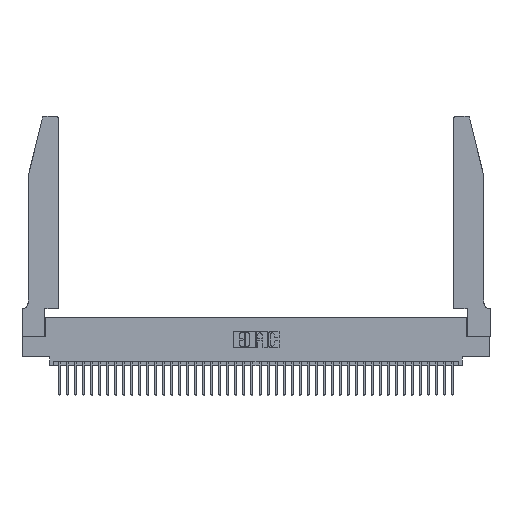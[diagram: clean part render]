
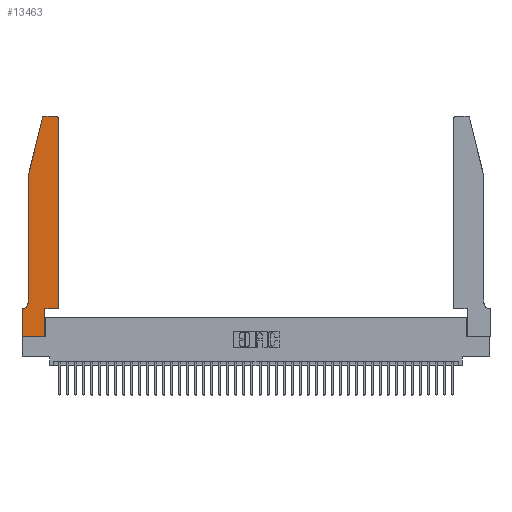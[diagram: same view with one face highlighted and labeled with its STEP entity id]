
A CAD part, top view. The second image highlights one B-rep face of the part: STEP entity #13463.
In plain terms, the highlighted planar face has unit normal (0, 0, 1).
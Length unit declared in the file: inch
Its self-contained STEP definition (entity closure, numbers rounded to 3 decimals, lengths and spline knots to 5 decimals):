
#49 = LINE ( 'NONE', #21602, #2139 ) ;
#389 = AXIS2_PLACEMENT_3D ( 'NONE', #16383, #23468, #19824 ) ;
#739 = CARTESIAN_POINT ( 'NONE',  ( 0.284, 2.75, 0.37 ) ) ;
#1626 = ORIENTED_EDGE ( 'NONE', *, *, #38126, .T. ) ;
#1852 = DIRECTION ( 'NONE',  ( 0., 1., 0. ) ) ;
#2139 = VECTOR ( 'NONE', #38475, 39.37008 ) ;
#2283 = EDGE_CURVE ( 'NONE', #10870, #23403, #25872, .T. ) ;
#2323 = VERTEX_POINT ( 'NONE', #41332 ) ;
#3364 = DIRECTION ( 'NONE',  ( 0., 0., 1. ) ) ;
#3447 = VECTOR ( 'NONE', #32906, 39.37008 ) ;
#3657 = CARTESIAN_POINT ( 'NONE',  ( 0.25487, 2.72718, 0.37 ) ) ;
#4674 = VERTEX_POINT ( 'NONE', #3657 ) ;
#5012 = AXIS2_PLACEMENT_3D ( 'NONE', #42519, #3364, #26780 ) ;
#5092 = EDGE_CURVE ( 'NONE', #36430, #42643, #23469, .T. ) ;
#5218 = EDGE_CURVE ( 'NONE', #23403, #35532, #49, .T. ) ;
#5223 = CARTESIAN_POINT ( 'NONE',  ( 0.4505, 0.35, 0.37 ) ) ;
#5322 = CARTESIAN_POINT ( 'NONE',  ( 0.2865, 0.35, 0.37 ) ) ;
#5338 = VERTEX_POINT ( 'NONE', #28809 ) ;
#5765 = ORIENTED_EDGE ( 'NONE', *, *, #24313, .T. ) ;
#5953 = EDGE_CURVE ( 'NONE', #5338, #42769, #11375, .T. ) ;
#6571 = CARTESIAN_POINT ( 'NONE',  ( 0.4505, 2.72, 0.37 ) ) ;
#6790 = CIRCLE ( 'NONE', #9981, 0.03 ) ;
#7419 = LINE ( 'NONE', #5223, #24640 ) ;
#8588 = CARTESIAN_POINT ( 'NONE',  ( 0.0755, 2., 0.37 ) ) ;
#8674 = VERTEX_POINT ( 'NONE', #6571 ) ;
#8936 = VERTEX_POINT ( 'NONE', #35670 ) ;
#9206 = ORIENTED_EDGE ( 'NONE', *, *, #5218, .T. ) ;
#9818 = VERTEX_POINT ( 'NONE', #5322 ) ;
#9981 = AXIS2_PLACEMENT_3D ( 'NONE', #21879, #14916, #18809 ) ;
#10870 = VERTEX_POINT ( 'NONE', #41445 ) ;
#11375 = LINE ( 'NONE', #18757, #33315 ) ;
#11379 = ORIENTED_EDGE ( 'NONE', *, *, #5092, .T. ) ;
#11959 = CARTESIAN_POINT ( 'NONE',  ( 0., 0., 0.37 ) ) ;
#12563 = ORIENTED_EDGE ( 'NONE', *, *, #35651, .T. ) ;
#13463 = ADVANCED_FACE ( 'NONE', ( #15908 ), #15897, .T. ) ;
#14860 = CIRCLE ( 'NONE', #389, 0.07 ) ;
#14861 = DIRECTION ( 'NONE',  ( -1., 0., 0. ) ) ;
#14916 = DIRECTION ( 'NONE',  ( 0., 0., 1. ) ) ;
#15897 = PLANE ( 'NONE',  #5012 ) ;
#15908 = FACE_OUTER_BOUND ( 'NONE', #16748, .T. ) ;
#16383 = CARTESIAN_POINT ( 'NONE',  ( 0.0055, 0.42, 0.37 ) ) ;
#16748 = EDGE_LOOP ( 'NONE', ( #27755, #1626, #18043, #11379, #16885, #33468, #38476, #9206, #23721, #37770, #5765, #12563 ) ) ;
#16885 = ORIENTED_EDGE ( 'NONE', *, *, #18688, .T. ) ;
#18039 = EDGE_CURVE ( 'NONE', #9818, #2323, #37777, .T. ) ;
#18043 = ORIENTED_EDGE ( 'NONE', *, *, #29669, .T. ) ;
#18110 = CARTESIAN_POINT ( 'NONE',  ( 0.284, 2.72, 0.37 ) ) ;
#18688 = EDGE_CURVE ( 'NONE', #42643, #8936, #14860, .T. ) ;
#18757 = CARTESIAN_POINT ( 'NONE',  ( 0.2605, 2.75, 0.37 ) ) ;
#18809 = DIRECTION ( 'NONE',  ( 1., 0., 0. ) ) ;
#19691 = CARTESIAN_POINT ( 'NONE',  ( 0., 0., 0.37 ) ) ;
#19752 = CARTESIAN_POINT ( 'NONE',  ( 0.4505, 0.35, 0.37 ) ) ;
#19824 = DIRECTION ( 'NONE',  ( -1., 0., 0. ) ) ;
#20065 = LINE ( 'NONE', #42934, #41975 ) ;
#20245 = LINE ( 'NONE', #29041, #25525 ) ;
#20588 = VECTOR ( 'NONE', #42229, 39.37008 ) ;
#21602 = CARTESIAN_POINT ( 'NONE',  ( 0., 0., 0.37 ) ) ;
#21879 = CARTESIAN_POINT ( 'NONE',  ( 0.4205, 2.72, 0.37 ) ) ;
#22395 = EDGE_CURVE ( 'NONE', #35532, #9818, #20065, .T. ) ;
#22742 = CARTESIAN_POINT ( 'NONE',  ( 0.0755, 2., 0.37 ) ) ;
#23403 = VERTEX_POINT ( 'NONE', #19691 ) ;
#23468 = DIRECTION ( 'NONE',  ( 0., 0., -1. ) ) ;
#23469 = LINE ( 'NONE', #22742, #32917 ) ;
#23721 = ORIENTED_EDGE ( 'NONE', *, *, #22395, .T. ) ;
#24313 = EDGE_CURVE ( 'NONE', #2323, #8674, #7419, .T. ) ;
#24640 = VECTOR ( 'NONE', #1852, 39.37008 ) ;
#25094 = CARTESIAN_POINT ( 'NONE',  ( 0.0755, 0.35, 0.37 ) ) ;
#25525 = VECTOR ( 'NONE', #38422, 39.37008 ) ;
#25872 = LINE ( 'NONE', #11959, #20588 ) ;
#26640 = DIRECTION ( 'NONE',  ( 0., 1., 0. ) ) ;
#26780 = DIRECTION ( 'NONE',  ( 1., 0., 0. ) ) ;
#27755 = ORIENTED_EDGE ( 'NONE', *, *, #5953, .T. ) ;
#28809 = CARTESIAN_POINT ( 'NONE',  ( 0.4205, 2.75, 0.37 ) ) ;
#29041 = CARTESIAN_POINT ( 'NONE',  ( 0.0755, 2., 0.37 ) ) ;
#29197 = VECTOR ( 'NONE', #38152, 39.37008 ) ;
#29318 = CARTESIAN_POINT ( 'NONE',  ( 0.0755, 0.42, 0.37 ) ) ;
#29669 = EDGE_CURVE ( 'NONE', #4674, #36430, #20245, .T. ) ;
#31375 = CARTESIAN_POINT ( 'NONE',  ( 0.2865, 0., 0.37 ) ) ;
#32212 = CIRCLE ( 'NONE', #42674, 0.03 ) ;
#32418 = EDGE_CURVE ( 'NONE', #8936, #10870, #34968, .T. ) ;
#32906 = DIRECTION ( 'NONE',  ( 1., 0., 0. ) ) ;
#32917 = VECTOR ( 'NONE', #39173, 39.37008 ) ;
#33315 = VECTOR ( 'NONE', #14861, 39.37008 ) ;
#33468 = ORIENTED_EDGE ( 'NONE', *, *, #32418, .T. ) ;
#34968 = LINE ( 'NONE', #25094, #29197 ) ;
#35482 = DIRECTION ( 'NONE',  ( 1., 0., 0. ) ) ;
#35532 = VERTEX_POINT ( 'NONE', #31375 ) ;
#35651 = EDGE_CURVE ( 'NONE', #8674, #5338, #6790, .T. ) ;
#35670 = CARTESIAN_POINT ( 'NONE',  ( 0.0055, 0.35, 0.37 ) ) ;
#36430 = VERTEX_POINT ( 'NONE', #8588 ) ;
#37770 = ORIENTED_EDGE ( 'NONE', *, *, #18039, .T. ) ;
#37777 = LINE ( 'NONE', #19752, #3447 ) ;
#38126 = EDGE_CURVE ( 'NONE', #42769, #4674, #32212, .T. ) ;
#38152 = DIRECTION ( 'NONE',  ( -1., 0., 0. ) ) ;
#38422 = DIRECTION ( 'NONE',  ( -0.239, -0.971, 0. ) ) ;
#38475 = DIRECTION ( 'NONE',  ( 1., 0., 0. ) ) ;
#38476 = ORIENTED_EDGE ( 'NONE', *, *, #2283, .T. ) ;
#39173 = DIRECTION ( 'NONE',  ( 0., -1., 0. ) ) ;
#41332 = CARTESIAN_POINT ( 'NONE',  ( 0.4505, 0.35, 0.37 ) ) ;
#41394 = DIRECTION ( 'NONE',  ( 0., 0., 1. ) ) ;
#41445 = CARTESIAN_POINT ( 'NONE',  ( 0., 0.35, 0.37 ) ) ;
#41975 = VECTOR ( 'NONE', #26640, 39.37008 ) ;
#42229 = DIRECTION ( 'NONE',  ( 0., -1., 0. ) ) ;
#42519 = CARTESIAN_POINT ( 'NONE',  ( 0., 0.35, 0.37 ) ) ;
#42643 = VERTEX_POINT ( 'NONE', #29318 ) ;
#42674 = AXIS2_PLACEMENT_3D ( 'NONE', #18110, #41394, #35482 ) ;
#42769 = VERTEX_POINT ( 'NONE', #739 ) ;
#42934 = CARTESIAN_POINT ( 'NONE',  ( 0.2865, 0.35, 0.37 ) ) ;
